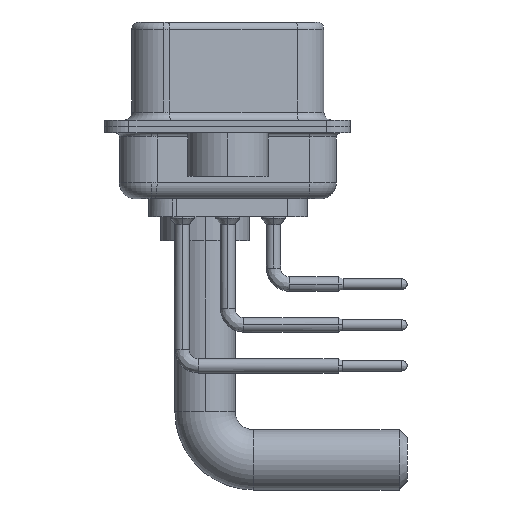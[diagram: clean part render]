
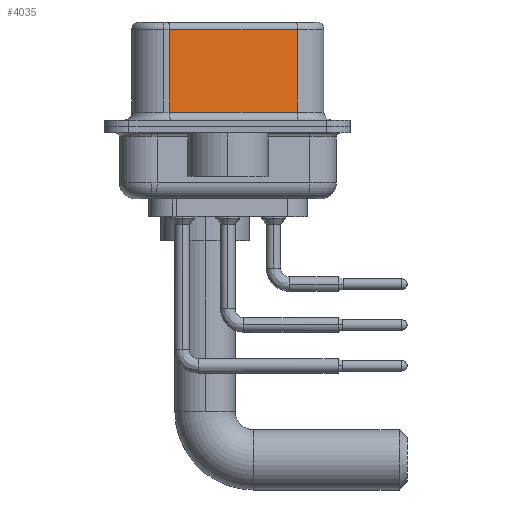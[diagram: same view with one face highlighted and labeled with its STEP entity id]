
A CAD part, left-side view. The second image highlights one B-rep face of the part: STEP entity #4035.
In plain terms, the highlighted planar face has unit normal (-0.985, -0.174, 0).
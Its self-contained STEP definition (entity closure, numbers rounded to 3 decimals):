
#3326 = CARTESIAN_POINT ( 'NONE',  ( 3.73, 3.628, 0.9 ) ) ;
#3990 = VERTEX_POINT ( 'NONE', #36210 ) ;
#4035 = ADVANCED_FACE ( 'NONE', ( #10335 ), #22261, .F. ) ;
#4474 = DIRECTION ( 'NONE',  ( 0., 0., -1. ) ) ;
#4548 = ORIENTED_EDGE ( 'NONE', *, *, #33650, .F. ) ;
#6521 = EDGE_CURVE ( 'NONE', #3990, #22111, #27620, .T. ) ;
#6958 = CARTESIAN_POINT ( 'NONE',  ( 5.132, -4.322, 6.02 ) ) ;
#7602 = ORIENTED_EDGE ( 'NONE', *, *, #6521, .T. ) ;
#7687 = EDGE_LOOP ( 'NONE', ( #4548, #26233, #7602, #19943 ) ) ;
#7797 = DIRECTION ( 'NONE',  ( 0., 0., -1. ) ) ;
#7970 = VECTOR ( 'NONE', #4474, 1000. ) ;
#8719 = VECTOR ( 'NONE', #35032, 1000. ) ;
#9879 = LINE ( 'NONE', #6958, #8719 ) ;
#10335 = FACE_OUTER_BOUND ( 'NONE', #7687, .T. ) ;
#10972 = CARTESIAN_POINT ( 'NONE',  ( 5.132, -4.322, 6.02 ) ) ;
#11045 = CARTESIAN_POINT ( 'NONE',  ( 5.132, -4.322, 6.52 ) ) ;
#12577 = VERTEX_POINT ( 'NONE', #10972 ) ;
#16532 = VERTEX_POINT ( 'NONE', #19957 ) ;
#17350 = CARTESIAN_POINT ( 'NONE',  ( 5.132, -4.322, 0.9 ) ) ;
#19943 = ORIENTED_EDGE ( 'NONE', *, *, #26898, .T. ) ;
#19957 = CARTESIAN_POINT ( 'NONE',  ( 5.132, -4.322, 0.9 ) ) ;
#22111 = VERTEX_POINT ( 'NONE', #3326 ) ;
#22261 = PLANE ( 'NONE',  #26427 ) ;
#22869 = VECTOR ( 'NONE', #25976, 1000. ) ;
#24220 = EDGE_CURVE ( 'NONE', #12577, #3990, #9879, .T. ) ;
#24289 = DIRECTION ( 'NONE',  ( -0.174, 0.985, 0. ) ) ;
#24733 = VECTOR ( 'NONE', #7797, 1000. ) ;
#25976 = DIRECTION ( 'NONE',  ( 0.174, -0.985, 0. ) ) ;
#26233 = ORIENTED_EDGE ( 'NONE', *, *, #24220, .T. ) ;
#26427 = AXIS2_PLACEMENT_3D ( 'NONE', #11045, #35857, #24289 ) ;
#26898 = EDGE_CURVE ( 'NONE', #22111, #16532, #28179, .T. ) ;
#27620 = LINE ( 'NONE', #36061, #24733 ) ;
#28179 = LINE ( 'NONE', #17350, #22869 ) ;
#32348 = CARTESIAN_POINT ( 'NONE',  ( 5.132, -4.322, 6.52 ) ) ;
#33650 = EDGE_CURVE ( 'NONE', #12577, #16532, #35646, .T. ) ;
#35032 = DIRECTION ( 'NONE',  ( -0.174, 0.985, 0. ) ) ;
#35646 = LINE ( 'NONE', #32348, #7970 ) ;
#35857 = DIRECTION ( 'NONE',  ( 0.985, 0.174, 0. ) ) ;
#36061 = CARTESIAN_POINT ( 'NONE',  ( 3.73, 3.628, 6.52 ) ) ;
#36210 = CARTESIAN_POINT ( 'NONE',  ( 3.73, 3.628, 6.02 ) ) ;
